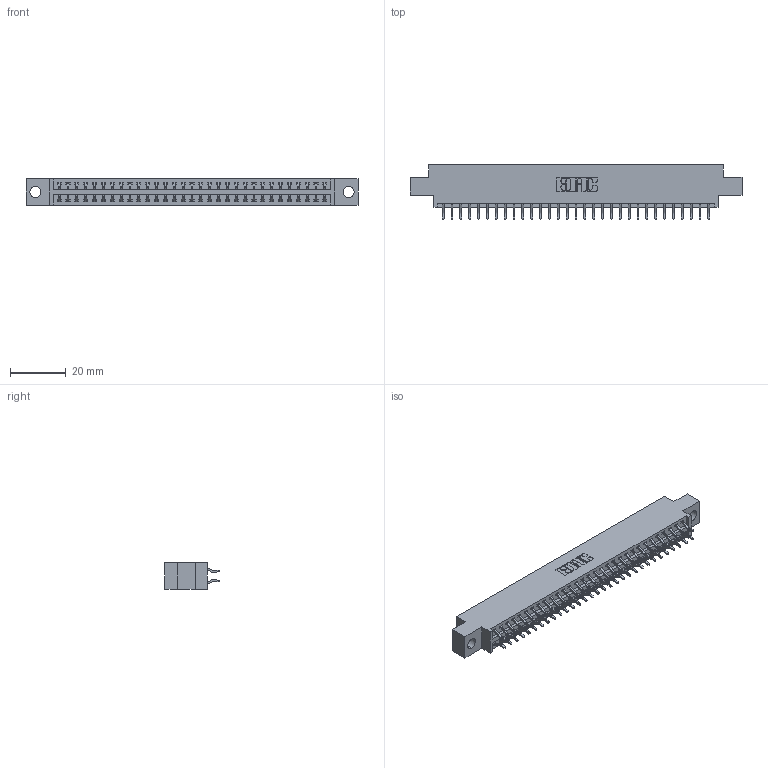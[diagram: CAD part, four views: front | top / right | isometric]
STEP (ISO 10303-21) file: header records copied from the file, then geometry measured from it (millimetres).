
FILE_DESCRIPTION (( 'STEP AP203' ), '1' );
FILE_NAME ('346-062-556-804.STEP', '2022-05-24T14:13:17', ( '' ), ( '' ), 'SwSTEP 2.0', 'SolidWorks 2020', '' );
FILE_SCHEMA (( 'CONFIG_CONTROL_DESIGN' ));
Length unit declared in the file: inch
Products named in the file (3): 346 Part_0.170 Offset - 0.156 Dia-TH; 346-062-556-804; 345-292-001_556 Tail
Assembly tree (63 placements, depth 2):
  346-062-556-804
    346 Part_0.170 Offset - 0.156 Dia-TH
    345-292-001_556 Tail  x62
Bounding box: 119 x 19.57 x 9.4 mm (x, y, z)
Volume: 11255.4 mm3; surface area: 15268.4 mm2
Topology: 63 solids, 63 shells, 3736 faces, 11103 edges, 7318 vertices
Faces by surface type: plane 2512, cylinder 1224
Entity records: 22483 total; most frequent: CARTESIAN_POINT 3742, ORIENTED_EDGE 3662, DIRECTION 3335, EDGE_CURVE 1831, VECTOR 1567, LINE 1567, VERTEX_POINT 1218, AXIS2_PLACEMENT_3D 884
